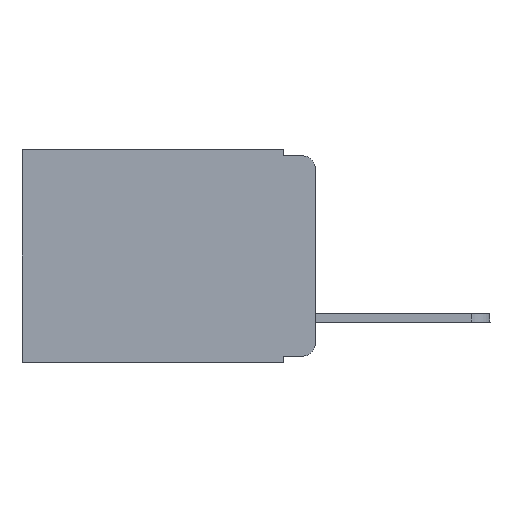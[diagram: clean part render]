
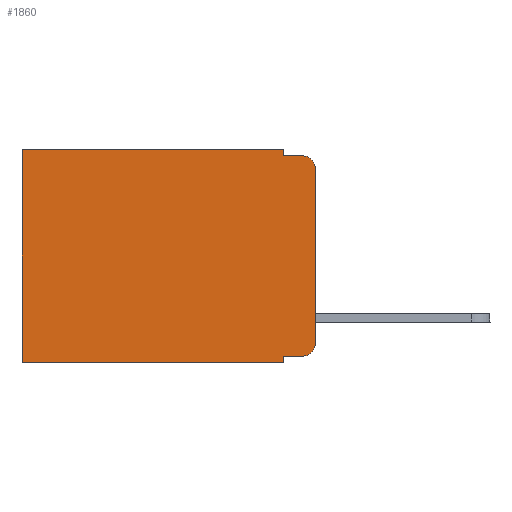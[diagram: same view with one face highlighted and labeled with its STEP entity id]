
A CAD part, left-side view. The second image highlights one B-rep face of the part: STEP entity #1860.
In plain terms, the highlighted planar face has unit normal (-1, 0, 0).
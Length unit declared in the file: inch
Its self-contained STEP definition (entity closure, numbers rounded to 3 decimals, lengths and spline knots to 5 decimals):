
#164 = FACE_OUTER_BOUND ( 'NONE', #11656, .T. ) ;
#216 = EDGE_CURVE ( 'NONE', #13353, #15690, #15333, .T. ) ;
#507 = CARTESIAN_POINT ( 'NONE',  ( 0.298, 0., -0.343 ) ) ;
#601 = CARTESIAN_POINT ( 'NONE',  ( 0.298, 0.051, 0. ) ) ;
#728 = CARTESIAN_POINT ( 'NONE',  ( 0.298, 0.473, 0. ) ) ;
#1090 = EDGE_CURVE ( 'NONE', #13353, #1936, #4830, .T. ) ;
#1251 = CARTESIAN_POINT ( 'NONE',  ( 0.298, 0.051, 0. ) ) ;
#1379 = AXIS2_PLACEMENT_3D ( 'NONE', #11769, #4959, #11832 ) ;
#1613 = VERTEX_POINT ( 'NONE', #13002 ) ;
#1756 = CARTESIAN_POINT ( 'NONE',  ( 0.298, 0.02, -0.313 ) ) ;
#1860 = ADVANCED_FACE ( 'NONE', ( #164 ), #7868, .F. ) ;
#1936 = VERTEX_POINT ( 'NONE', #13224 ) ;
#2774 = CARTESIAN_POINT ( 'NONE',  ( 0.298, 0., -0.03 ) ) ;
#2937 = EDGE_CURVE ( 'NONE', #1936, #8076, #12755, .T. ) ;
#3191 = ORIENTED_EDGE ( 'NONE', *, *, #16113, .F. ) ;
#3259 = DIRECTION ( 'NONE',  ( 0., 0., -1. ) ) ;
#3486 = CARTESIAN_POINT ( 'NONE',  ( 0.298, 0.02, -0.03 ) ) ;
#3514 = EDGE_CURVE ( 'NONE', #8844, #5217, #8337, .T. ) ;
#3823 = CARTESIAN_POINT ( 'NONE',  ( 0.298, 0.051, 0. ) ) ;
#3892 = CARTESIAN_POINT ( 'NONE',  ( 0.298, 0., 0. ) ) ;
#3933 = VECTOR ( 'NONE', #15228, 39.37008 ) ;
#3992 = VECTOR ( 'NONE', #3259, 39.37008 ) ;
#4057 = ORIENTED_EDGE ( 'NONE', *, *, #8704, .F. ) ;
#4255 = EDGE_CURVE ( 'NONE', #8844, #4763, #9145, .T. ) ;
#4557 = DIRECTION ( 'NONE',  ( 0., -1., 0. ) ) ;
#4763 = VERTEX_POINT ( 'NONE', #9546 ) ;
#4830 = LINE ( 'NONE', #601, #3992 ) ;
#4850 = VECTOR ( 'NONE', #7532, 39.37008 ) ;
#4959 = DIRECTION ( 'NONE',  ( 1., 0., 0. ) ) ;
#5159 = DIRECTION ( 'NONE',  ( 0., 0., -1. ) ) ;
#5217 = VERTEX_POINT ( 'NONE', #9091 ) ;
#5219 = CARTESIAN_POINT ( 'NONE',  ( 0.298, 0., 0. ) ) ;
#6024 = ORIENTED_EDGE ( 'NONE', *, *, #10887, .T. ) ;
#7496 = VECTOR ( 'NONE', #12050, 39.37008 ) ;
#7503 = ORIENTED_EDGE ( 'NONE', *, *, #7634, .T. ) ;
#7532 = DIRECTION ( 'NONE',  ( 0., -1., 0. ) ) ;
#7573 = ORIENTED_EDGE ( 'NONE', *, *, #13161, .T. ) ;
#7634 = EDGE_CURVE ( 'NONE', #13460, #14564, #10946, .T. ) ;
#7674 = LINE ( 'NONE', #16671, #12538 ) ;
#7709 = CARTESIAN_POINT ( 'NONE',  ( 0.298, 0.051, -0.333 ) ) ;
#7868 = PLANE ( 'NONE',  #1379 ) ;
#8076 = VERTEX_POINT ( 'NONE', #12986 ) ;
#8337 = LINE ( 'NONE', #3892, #7496 ) ;
#8462 = CIRCLE ( 'NONE', #12939, 0.02 ) ;
#8704 = EDGE_CURVE ( 'NONE', #13460, #1613, #14897, .T. ) ;
#8844 = VERTEX_POINT ( 'NONE', #2774 ) ;
#9091 = CARTESIAN_POINT ( 'NONE',  ( 0.298, 0., -0.313 ) ) ;
#9145 = CIRCLE ( 'NONE', #11179, 0.02 ) ;
#9546 = CARTESIAN_POINT ( 'NONE',  ( 0.298, 0.02, -0.01 ) ) ;
#10275 = VECTOR ( 'NONE', #5159, 39.37008 ) ;
#10887 = EDGE_CURVE ( 'NONE', #14564, #8076, #16272, .T. ) ;
#10946 = LINE ( 'NONE', #5219, #13023 ) ;
#11131 = DIRECTION ( 'NONE',  ( -1., 0., 0. ) ) ;
#11179 = AXIS2_PLACEMENT_3D ( 'NONE', #3486, #11407, #16982 ) ;
#11407 = DIRECTION ( 'NONE',  ( -1., 0., 0. ) ) ;
#11656 = EDGE_LOOP ( 'NONE', ( #16886, #15571, #3191, #4057, #7503, #6024, #12292, #12165, #16318, #7573 ) ) ;
#11769 = CARTESIAN_POINT ( 'NONE',  ( 0.298, 0., 0. ) ) ;
#11832 = DIRECTION ( 'NONE',  ( 0., 0., -1. ) ) ;
#12050 = DIRECTION ( 'NONE',  ( 0., 0., -1. ) ) ;
#12165 = ORIENTED_EDGE ( 'NONE', *, *, #1090, .F. ) ;
#12292 = ORIENTED_EDGE ( 'NONE', *, *, #2937, .F. ) ;
#12538 = VECTOR ( 'NONE', #4557, 39.37008 ) ;
#12755 = LINE ( 'NONE', #507, #3933 ) ;
#12857 = CARTESIAN_POINT ( 'NONE',  ( 0.298, 0.02, -0.333 ) ) ;
#12939 = AXIS2_PLACEMENT_3D ( 'NONE', #1756, #11131, #13875 ) ;
#12986 = CARTESIAN_POINT ( 'NONE',  ( 0.298, 0.473, -0.343 ) ) ;
#13002 = CARTESIAN_POINT ( 'NONE',  ( 0.298, 0.051, -0.01 ) ) ;
#13023 = VECTOR ( 'NONE', #13264, 39.37008 ) ;
#13161 = EDGE_CURVE ( 'NONE', #15690, #5217, #8462, .T. ) ;
#13224 = CARTESIAN_POINT ( 'NONE',  ( 0.298, 0.051, -0.343 ) ) ;
#13242 = DIRECTION ( 'NONE',  ( 0., 0., -1. ) ) ;
#13264 = DIRECTION ( 'NONE',  ( 0., 1., 0. ) ) ;
#13353 = VERTEX_POINT ( 'NONE', #17169 ) ;
#13460 = VERTEX_POINT ( 'NONE', #1251 ) ;
#13875 = DIRECTION ( 'NONE',  ( 0., 0., -1. ) ) ;
#14191 = VECTOR ( 'NONE', #13242, 39.37008 ) ;
#14564 = VERTEX_POINT ( 'NONE', #728 ) ;
#14897 = LINE ( 'NONE', #3823, #10275 ) ;
#15228 = DIRECTION ( 'NONE',  ( 0., 1., 0. ) ) ;
#15333 = LINE ( 'NONE', #7709, #4850 ) ;
#15571 = ORIENTED_EDGE ( 'NONE', *, *, #4255, .T. ) ;
#15690 = VERTEX_POINT ( 'NONE', #12857 ) ;
#15861 = CARTESIAN_POINT ( 'NONE',  ( 0.298, 0.473, 0. ) ) ;
#16113 = EDGE_CURVE ( 'NONE', #1613, #4763, #7674, .T. ) ;
#16272 = LINE ( 'NONE', #15861, #14191 ) ;
#16318 = ORIENTED_EDGE ( 'NONE', *, *, #216, .T. ) ;
#16671 = CARTESIAN_POINT ( 'NONE',  ( 0.298, 0.051, -0.01 ) ) ;
#16886 = ORIENTED_EDGE ( 'NONE', *, *, #3514, .F. ) ;
#16982 = DIRECTION ( 'NONE',  ( 0., 0., -1. ) ) ;
#17169 = CARTESIAN_POINT ( 'NONE',  ( 0.298, 0.051, -0.333 ) ) ;
